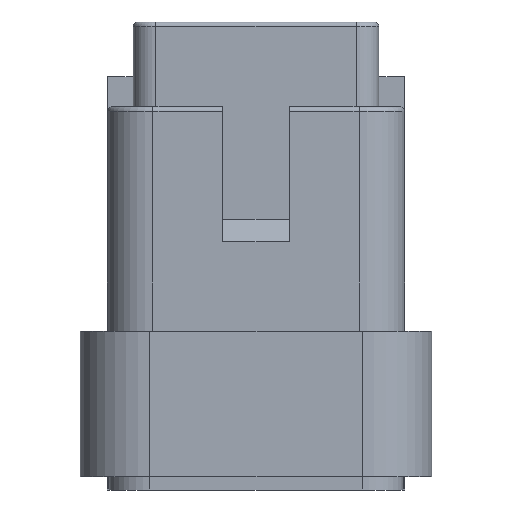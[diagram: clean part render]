
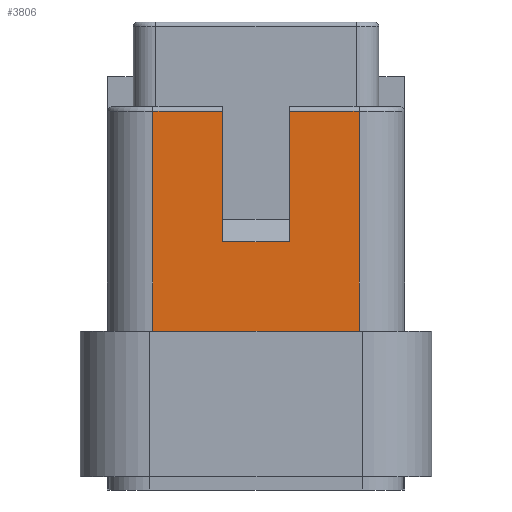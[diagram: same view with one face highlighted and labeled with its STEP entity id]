
A CAD part, front view. The second image highlights one B-rep face of the part: STEP entity #3806.
In plain terms, the highlighted planar face has unit normal (0, -1, 0).
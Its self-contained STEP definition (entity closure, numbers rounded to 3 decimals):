
#128 = ORIENTED_EDGE ( 'NONE', *, *, #2117, .T. ) ;
#470 = VECTOR ( 'NONE', #2890, 1000. ) ;
#609 = CARTESIAN_POINT ( 'NONE',  ( 0.65, -0.75, -10.2 ) ) ;
#840 = DIRECTION ( 'NONE',  ( 0., 0., 1. ) ) ;
#1270 = VECTOR ( 'NONE', #10766, 1000. ) ;
#1290 = EDGE_CURVE ( 'NONE', #3703, #5908, #10796, .T. ) ;
#2069 = VECTOR ( 'NONE', #9706, 1000. ) ;
#2108 = ORIENTED_EDGE ( 'NONE', *, *, #1290, .T. ) ;
#2117 = EDGE_CURVE ( 'NONE', #11256, #7795, #8741, .T. ) ;
#2288 = ORIENTED_EDGE ( 'NONE', *, *, #3833, .T. ) ;
#2403 = ORIENTED_EDGE ( 'NONE', *, *, #3313, .F. ) ;
#2544 = CARTESIAN_POINT ( 'NONE',  ( 5.15, -0.75, -2.95 ) ) ;
#2890 = DIRECTION ( 'NONE',  ( 0., 0., 1. ) ) ;
#2961 = ORIENTED_EDGE ( 'NONE', *, *, #9927, .F. ) ;
#2993 = ORIENTED_EDGE ( 'NONE', *, *, #11788, .T. ) ;
#3313 = EDGE_CURVE ( 'NONE', #6064, #7409, #11769, .T. ) ;
#3574 = CARTESIAN_POINT ( 'NONE',  ( 7.45, -0.75, -10.2 ) ) ;
#3703 = VERTEX_POINT ( 'NONE', #3574 ) ;
#3761 = LINE ( 'NONE', #10682, #2069 ) ;
#3806 = ADVANCED_FACE ( 'NONE', ( #6663 ), #5882, .F. ) ;
#3833 = EDGE_CURVE ( 'NONE', #6064, #11256, #3761, .T. ) ;
#3839 = CARTESIAN_POINT ( 'NONE',  ( 2.95, -0.75, -6.4 ) ) ;
#4822 = LINE ( 'NONE', #8749, #470 ) ;
#5034 = CARTESIAN_POINT ( 'NONE',  ( 7.45, -0.75, -10.2 ) ) ;
#5391 = DIRECTION ( 'NONE',  ( -1., 0., 0. ) ) ;
#5397 = VECTOR ( 'NONE', #10986, 1000. ) ;
#5812 = CARTESIAN_POINT ( 'NONE',  ( 7.45, -0.75, -2.95 ) ) ;
#5882 = PLANE ( 'NONE',  #9866 ) ;
#5908 = VERTEX_POINT ( 'NONE', #5812 ) ;
#5960 = CARTESIAN_POINT ( 'NONE',  ( 5.15, -0.75, -6.4 ) ) ;
#6064 = VERTEX_POINT ( 'NONE', #8902 ) ;
#6097 = VECTOR ( 'NONE', #9374, 1000. ) ;
#6663 = FACE_OUTER_BOUND ( 'NONE', #7317, .T. ) ;
#6877 = CARTESIAN_POINT ( 'NONE',  ( 2.95, -0.75, -2.95 ) ) ;
#7317 = EDGE_LOOP ( 'NONE', ( #2108, #9720, #2403, #2288, #128, #2993, #8685, #2961 ) ) ;
#7409 = VERTEX_POINT ( 'NONE', #9801 ) ;
#7727 = EDGE_CURVE ( 'NONE', #10934, #10379, #4822, .T. ) ;
#7752 = CARTESIAN_POINT ( 'NONE',  ( 7.45, -0.75, -10.2 ) ) ;
#7795 = VERTEX_POINT ( 'NONE', #6877 ) ;
#8151 = LINE ( 'NONE', #10294, #10877 ) ;
#8326 = VECTOR ( 'NONE', #10194, 1000. ) ;
#8330 = LINE ( 'NONE', #2544, #6097 ) ;
#8685 = ORIENTED_EDGE ( 'NONE', *, *, #7727, .F. ) ;
#8741 = LINE ( 'NONE', #3839, #9080 ) ;
#8749 = CARTESIAN_POINT ( 'NONE',  ( 0.65, -0.75, -10.2 ) ) ;
#8902 = CARTESIAN_POINT ( 'NONE',  ( 5.15, -0.75, -7.25 ) ) ;
#9080 = VECTOR ( 'NONE', #11701, 1000. ) ;
#9146 = CARTESIAN_POINT ( 'NONE',  ( 0.65, -0.75, -2.95 ) ) ;
#9372 = EDGE_CURVE ( 'NONE', #5908, #7409, #8330, .T. ) ;
#9374 = DIRECTION ( 'NONE',  ( -1., 0., 0. ) ) ;
#9706 = DIRECTION ( 'NONE',  ( -1., 0., 0. ) ) ;
#9720 = ORIENTED_EDGE ( 'NONE', *, *, #9372, .T. ) ;
#9801 = CARTESIAN_POINT ( 'NONE',  ( 5.15, -0.75, -2.95 ) ) ;
#9832 = DIRECTION ( 'NONE',  ( 0., 1., 0. ) ) ;
#9866 = AXIS2_PLACEMENT_3D ( 'NONE', #7752, #9832, #840 ) ;
#9927 = EDGE_CURVE ( 'NONE', #3703, #10934, #8151, .T. ) ;
#10194 = DIRECTION ( 'NONE',  ( -1., 0., 0. ) ) ;
#10294 = CARTESIAN_POINT ( 'NONE',  ( 7.45, -0.75, -10.2 ) ) ;
#10379 = VERTEX_POINT ( 'NONE', #12455 ) ;
#10682 = CARTESIAN_POINT ( 'NONE',  ( 2.95, -0.75, -7.25 ) ) ;
#10766 = DIRECTION ( 'NONE',  ( 0., 0., 1. ) ) ;
#10796 = LINE ( 'NONE', #5034, #5397 ) ;
#10877 = VECTOR ( 'NONE', #5391, 1000. ) ;
#10934 = VERTEX_POINT ( 'NONE', #609 ) ;
#10972 = LINE ( 'NONE', #9146, #8326 ) ;
#10986 = DIRECTION ( 'NONE',  ( 0., 0., 1. ) ) ;
#11256 = VERTEX_POINT ( 'NONE', #11825 ) ;
#11701 = DIRECTION ( 'NONE',  ( 0., 0., 1. ) ) ;
#11769 = LINE ( 'NONE', #5960, #1270 ) ;
#11788 = EDGE_CURVE ( 'NONE', #7795, #10379, #10972, .T. ) ;
#11825 = CARTESIAN_POINT ( 'NONE',  ( 2.95, -0.75, -7.25 ) ) ;
#12455 = CARTESIAN_POINT ( 'NONE',  ( 0.65, -0.75, -2.95 ) ) ;
